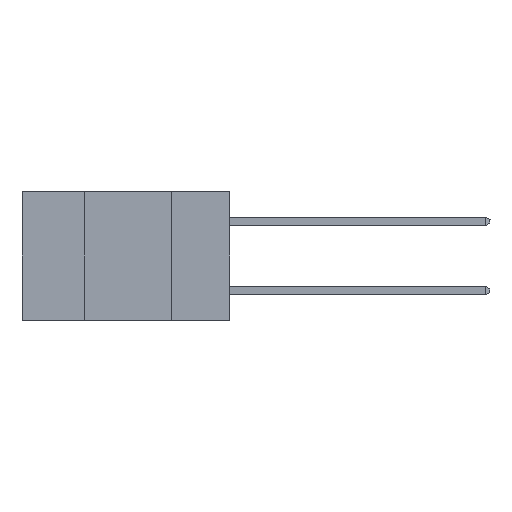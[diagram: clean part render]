
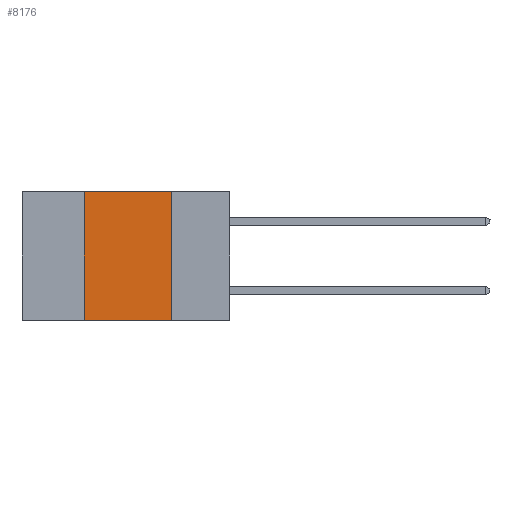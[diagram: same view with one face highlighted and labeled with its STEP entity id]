
A CAD part, left-side view. The second image highlights one B-rep face of the part: STEP entity #8176.
In plain terms, the highlighted planar face has unit normal (-1, 0, 0).
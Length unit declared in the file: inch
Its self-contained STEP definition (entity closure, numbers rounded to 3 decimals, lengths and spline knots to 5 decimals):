
#67 = CARTESIAN_POINT ( 'NONE',  ( 0., 0.17, -0.37 ) ) ;
#1160 = VECTOR ( 'NONE', #9321, 39.37008 ) ;
#1537 = LINE ( 'NONE', #4627, #17492 ) ;
#2062 = CARTESIAN_POINT ( 'NONE',  ( 0., 0.6, 0. ) ) ;
#2260 = VECTOR ( 'NONE', #5238, 39.37008 ) ;
#2540 = LINE ( 'NONE', #13948, #2260 ) ;
#4027 = DIRECTION ( 'NONE',  ( 0., 0., -1. ) ) ;
#4111 = AXIS2_PLACEMENT_3D ( 'NONE', #5573, #8497, #4027 ) ;
#4610 = CARTESIAN_POINT ( 'NONE',  ( 0., 0.17, -0.37 ) ) ;
#4627 = CARTESIAN_POINT ( 'NONE',  ( 0., 0.6, -0.37 ) ) ;
#4943 = ORIENTED_EDGE ( 'NONE', *, *, #10102, .F. ) ;
#5238 = DIRECTION ( 'NONE',  ( 0., 0., 1. ) ) ;
#5573 = CARTESIAN_POINT ( 'NONE',  ( 0., 0.6, 0. ) ) ;
#6308 = LINE ( 'NONE', #2062, #1160 ) ;
#6587 = EDGE_LOOP ( 'NONE', ( #8502, #13666, #4943, #7259 ) ) ;
#6651 = VERTEX_POINT ( 'NONE', #4610 ) ;
#7014 = CARTESIAN_POINT ( 'NONE',  ( 0., 0.17, 0. ) ) ;
#7259 = ORIENTED_EDGE ( 'NONE', *, *, #13965, .T. ) ;
#7856 = EDGE_CURVE ( 'NONE', #18818, #6651, #14872, .T. ) ;
#8176 = ADVANCED_FACE ( 'NONE', ( #8594 ), #15845, .F. ) ;
#8497 = DIRECTION ( 'NONE',  ( 1., 0., 0. ) ) ;
#8502 = ORIENTED_EDGE ( 'NONE', *, *, #7856, .F. ) ;
#8594 = FACE_OUTER_BOUND ( 'NONE', #6587, .T. ) ;
#8821 = CARTESIAN_POINT ( 'NONE',  ( 0., 0.42, -0.37 ) ) ;
#9321 = DIRECTION ( 'NONE',  ( 0., -1., 0. ) ) ;
#9383 = VERTEX_POINT ( 'NONE', #10157 ) ;
#10102 = EDGE_CURVE ( 'NONE', #17162, #9383, #2540, .T. ) ;
#10157 = CARTESIAN_POINT ( 'NONE',  ( 0., 0.42, 0. ) ) ;
#13666 = ORIENTED_EDGE ( 'NONE', *, *, #16946, .F. ) ;
#13948 = CARTESIAN_POINT ( 'NONE',  ( 0., 0.42, -0.37 ) ) ;
#13965 = EDGE_CURVE ( 'NONE', #17162, #6651, #1537, .T. ) ;
#14776 = DIRECTION ( 'NONE',  ( 0., 0., -1. ) ) ;
#14872 = LINE ( 'NONE', #67, #17692 ) ;
#14972 = DIRECTION ( 'NONE',  ( 0., -1., 0. ) ) ;
#15845 = PLANE ( 'NONE',  #4111 ) ;
#16946 = EDGE_CURVE ( 'NONE', #9383, #18818, #6308, .T. ) ;
#17162 = VERTEX_POINT ( 'NONE', #8821 ) ;
#17492 = VECTOR ( 'NONE', #14972, 39.37008 ) ;
#17692 = VECTOR ( 'NONE', #14776, 39.37008 ) ;
#18818 = VERTEX_POINT ( 'NONE', #7014 ) ;
